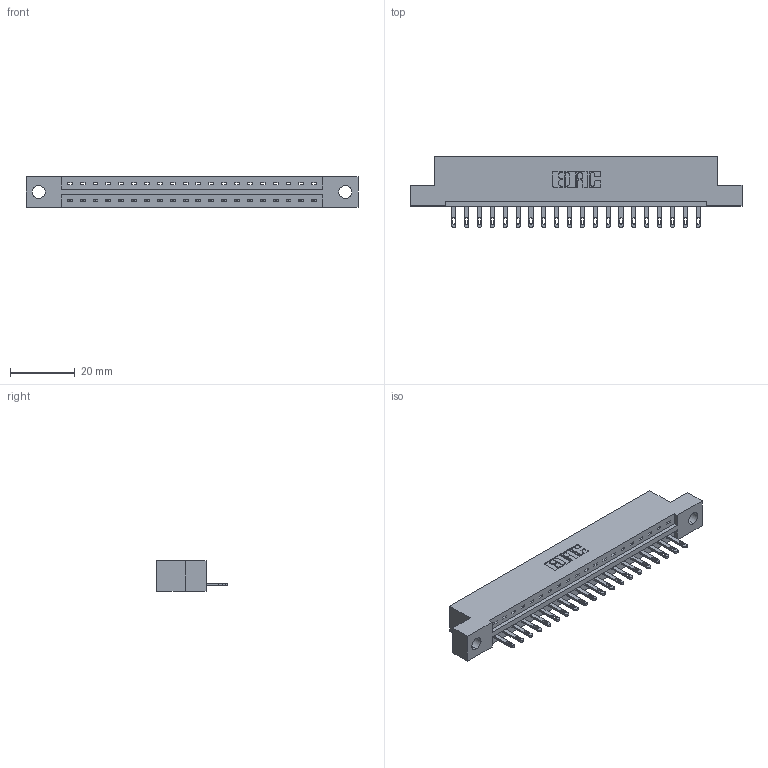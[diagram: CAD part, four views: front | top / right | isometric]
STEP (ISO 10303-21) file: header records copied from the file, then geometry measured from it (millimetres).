
FILE_DESCRIPTION (( 'STEP AP203' ), '1' );
FILE_NAME ('337-020-500-104.STEP', '2018-08-05T07:55:02', ( '' ), ( '' ), 'SwSTEP 2.0', 'SolidWorks 2016', '' );
FILE_SCHEMA (( 'CONFIG_CONTROL_DESIGN' ));
Length unit declared in the file: inch
Products named in the file (3): 337 Part_Flush Mounting Lugs - 0.156 Dia-TH; 345-292-001_345-293-100; 337-020-500-104
Assembly tree (21 placements, depth 2):
  337-020-500-104
    337 Part_Flush Mounting Lugs - 0.156 Dia-TH
    345-292-001_345-293-100  x20
Bounding box: 102.26 x 21.85 x 9.4 mm (x, y, z)
Volume: 10277.5 mm3; surface area: 10340.1 mm2
Topology: 21 solids, 21 shells, 1274 faces, 3911 edges, 2606 vertices
Faces by surface type: plane 870, cylinder 404
Entity records: 17645 total; most frequent: CARTESIAN_POINT 3078, ORIENTED_EDGE 3034, DIRECTION 2637, EDGE_CURVE 1517, LINE 1385, VECTOR 1385, VERTEX_POINT 1010, AXIS2_PLACEMENT_3D 626
